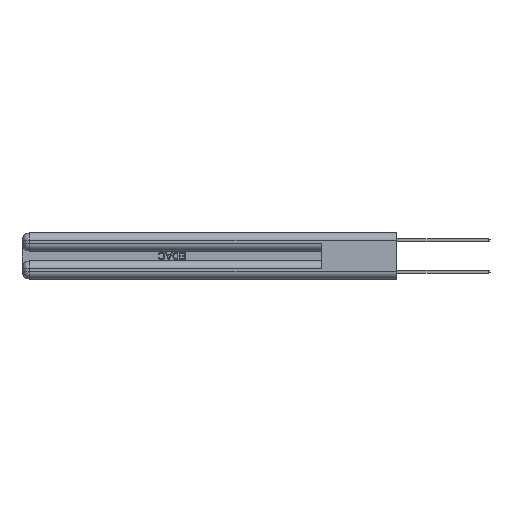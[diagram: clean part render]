
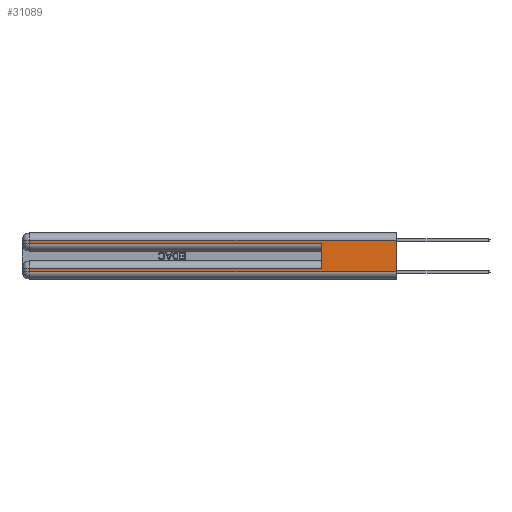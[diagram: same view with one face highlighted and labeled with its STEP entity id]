
A CAD part, left-side view. The second image highlights one B-rep face of the part: STEP entity #31089.
In plain terms, the highlighted planar face has unit normal (-1, 0, 0).
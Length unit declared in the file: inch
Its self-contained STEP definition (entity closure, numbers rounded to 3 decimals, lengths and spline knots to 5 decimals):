
#535 = VECTOR ( 'NONE', #19135, 39.37008 ) ;
#665 = EDGE_CURVE ( 'NONE', #22211, #4428, #31676, .T. ) ;
#1092 = CARTESIAN_POINT ( 'NONE',  ( 0., 0., 0.06 ) ) ;
#1283 = EDGE_CURVE ( 'NONE', #17996, #2534, #26491, .T. ) ;
#1807 = VERTEX_POINT ( 'NONE', #23907 ) ;
#1864 = ORIENTED_EDGE ( 'NONE', *, *, #26216, .T. ) ;
#2235 = VECTOR ( 'NONE', #14873, 39.37008 ) ;
#2534 = VERTEX_POINT ( 'NONE', #6470 ) ;
#2579 = DIRECTION ( 'NONE',  ( 0., 1., 0. ) ) ;
#3032 = EDGE_CURVE ( 'NONE', #3314, #2534, #3582, .T. ) ;
#3314 = VERTEX_POINT ( 'NONE', #6670 ) ;
#3582 = LINE ( 'NONE', #1092, #535 ) ;
#4428 = VERTEX_POINT ( 'NONE', #20471 ) ;
#4886 = VERTEX_POINT ( 'NONE', #25782 ) ;
#5976 = ORIENTED_EDGE ( 'NONE', *, *, #3032, .T. ) ;
#6470 = CARTESIAN_POINT ( 'NONE',  ( 0., 0., 0.06 ) ) ;
#6670 = CARTESIAN_POINT ( 'NONE',  ( 0., 2.94, 0.06 ) ) ;
#6873 = EDGE_LOOP ( 'NONE', ( #24362, #32168, #9527, #19841, #13749, #1864, #21048, #5976 ) ) ;
#7954 = EDGE_CURVE ( 'NONE', #17996, #11249, #23306, .T. ) ;
#8326 = VECTOR ( 'NONE', #2579, 39.37008 ) ;
#9527 = ORIENTED_EDGE ( 'NONE', *, *, #21373, .T. ) ;
#10664 = EDGE_CURVE ( 'NONE', #4886, #3314, #13993, .T. ) ;
#11249 = VERTEX_POINT ( 'NONE', #17272 ) ;
#13749 = ORIENTED_EDGE ( 'NONE', *, *, #665, .F. ) ;
#13911 = LINE ( 'NONE', #26773, #28796 ) ;
#13993 = LINE ( 'NONE', #24183, #30883 ) ;
#14513 = CARTESIAN_POINT ( 'NONE',  ( 0., 0.6, 0.085 ) ) ;
#14873 = DIRECTION ( 'NONE',  ( 0., -1., 0. ) ) ;
#15340 = CARTESIAN_POINT ( 'NONE',  ( 0., 0., 0.31 ) ) ;
#15630 = DIRECTION ( 'NONE',  ( 0., 0., -1. ) ) ;
#16185 = DIRECTION ( 'NONE',  ( 1., 0., 0. ) ) ;
#16286 = CARTESIAN_POINT ( 'NONE',  ( 0., 0., 0.37 ) ) ;
#16635 = CARTESIAN_POINT ( 'NONE',  ( 0., 2.94, 0.37 ) ) ;
#16730 = DIRECTION ( 'NONE',  ( 0., 1., 0. ) ) ;
#16958 = LINE ( 'NONE', #16635, #26414 ) ;
#17272 = CARTESIAN_POINT ( 'NONE',  ( 0., 2.94, 0.31 ) ) ;
#17453 = CARTESIAN_POINT ( 'NONE',  ( 0., 0., 0.31 ) ) ;
#17996 = VERTEX_POINT ( 'NONE', #15340 ) ;
#18762 = CARTESIAN_POINT ( 'NONE',  ( 0., 0.6, 0.145 ) ) ;
#18999 = EDGE_CURVE ( 'NONE', #1807, #4428, #29756, .T. ) ;
#19011 = DIRECTION ( 'NONE',  ( 0., 0., -1. ) ) ;
#19135 = DIRECTION ( 'NONE',  ( 0., -1., 0. ) ) ;
#19841 = ORIENTED_EDGE ( 'NONE', *, *, #18999, .T. ) ;
#20471 = CARTESIAN_POINT ( 'NONE',  ( 0., 0.6, 0.285 ) ) ;
#21048 = ORIENTED_EDGE ( 'NONE', *, *, #10664, .T. ) ;
#21373 = EDGE_CURVE ( 'NONE', #11249, #1807, #16958, .T. ) ;
#22211 = VERTEX_POINT ( 'NONE', #14513 ) ;
#23306 = LINE ( 'NONE', #17453, #8326 ) ;
#23907 = CARTESIAN_POINT ( 'NONE',  ( 0., 2.94, 0.285 ) ) ;
#24183 = CARTESIAN_POINT ( 'NONE',  ( 0., 2.94, 0.37 ) ) ;
#24362 = ORIENTED_EDGE ( 'NONE', *, *, #1283, .F. ) ;
#25782 = CARTESIAN_POINT ( 'NONE',  ( 0., 2.94, 0.085 ) ) ;
#25863 = VECTOR ( 'NONE', #15630, 39.37008 ) ;
#25885 = CARTESIAN_POINT ( 'NONE',  ( 0., 0., 0.37 ) ) ;
#26216 = EDGE_CURVE ( 'NONE', #22211, #4886, #13911, .T. ) ;
#26414 = VECTOR ( 'NONE', #31896, 39.37008 ) ;
#26491 = LINE ( 'NONE', #16286, #25863 ) ;
#26773 = CARTESIAN_POINT ( 'NONE',  ( 0., 0., 0.085 ) ) ;
#28796 = VECTOR ( 'NONE', #16730, 39.37008 ) ;
#28914 = FACE_OUTER_BOUND ( 'NONE', #6873, .T. ) ;
#28975 = DIRECTION ( 'NONE',  ( 0., 0., 1. ) ) ;
#29228 = VECTOR ( 'NONE', #28975, 39.37008 ) ;
#29392 = DIRECTION ( 'NONE',  ( 0., 0., -1. ) ) ;
#29756 = LINE ( 'NONE', #32447, #2235 ) ;
#30547 = AXIS2_PLACEMENT_3D ( 'NONE', #25885, #16185, #19011 ) ;
#30883 = VECTOR ( 'NONE', #29392, 39.37008 ) ;
#31089 = ADVANCED_FACE ( 'NONE', ( #28914 ), #31272, .F. ) ;
#31272 = PLANE ( 'NONE',  #30547 ) ;
#31676 = LINE ( 'NONE', #18762, #29228 ) ;
#31896 = DIRECTION ( 'NONE',  ( 0., 0., -1. ) ) ;
#32168 = ORIENTED_EDGE ( 'NONE', *, *, #7954, .T. ) ;
#32447 = CARTESIAN_POINT ( 'NONE',  ( 0., 0., 0.285 ) ) ;
